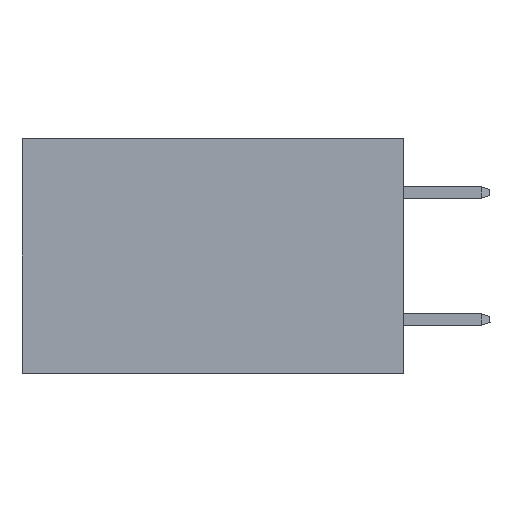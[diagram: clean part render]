
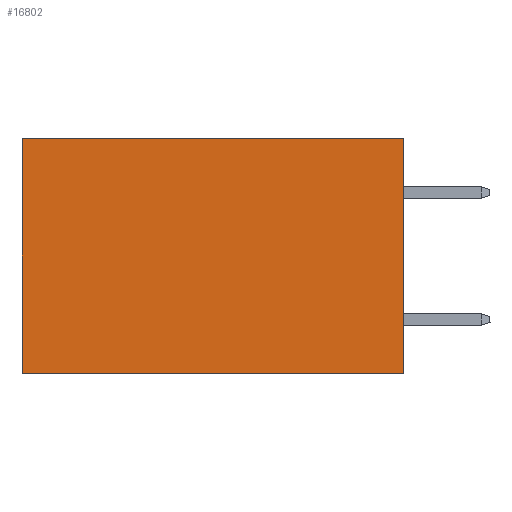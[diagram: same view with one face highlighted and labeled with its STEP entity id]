
A CAD part, left-side view. The second image highlights one B-rep face of the part: STEP entity #16802.
In plain terms, the highlighted planar face has unit normal (-1, 0, 0).
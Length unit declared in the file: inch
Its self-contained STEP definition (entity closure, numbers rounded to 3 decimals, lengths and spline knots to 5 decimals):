
#21 = VECTOR ( 'NONE', #15168, 39.37008 ) ;
#228 = EDGE_CURVE ( 'NONE', #13715, #8388, #10651, .T. ) ;
#1022 = CARTESIAN_POINT ( 'NONE',  ( 0.2875, 0., 0. ) ) ;
#2741 = EDGE_CURVE ( 'NONE', #18579, #13715, #11889, .T. ) ;
#2915 = AXIS2_PLACEMENT_3D ( 'NONE', #3194, #5733, #23075 ) ;
#3194 = CARTESIAN_POINT ( 'NONE',  ( 0.2875, 0., 0. ) ) ;
#3253 = ORIENTED_EDGE ( 'NONE', *, *, #4046, .F. ) ;
#3338 = FACE_OUTER_BOUND ( 'NONE', #24918, .T. ) ;
#4046 = EDGE_CURVE ( 'NONE', #18579, #14857, #15443, .T. ) ;
#5733 = DIRECTION ( 'NONE',  ( 1., 0., 0. ) ) ;
#6467 = DIRECTION ( 'NONE',  ( 0., 0., -1. ) ) ;
#7095 = VECTOR ( 'NONE', #24897, 39.37008 ) ;
#7417 = LINE ( 'NONE', #24339, #7095 ) ;
#8388 = VERTEX_POINT ( 'NONE', #27807 ) ;
#8551 = ORIENTED_EDGE ( 'NONE', *, *, #2741, .T. ) ;
#10651 = LINE ( 'NONE', #15074, #17989 ) ;
#11889 = LINE ( 'NONE', #14150, #18251 ) ;
#13335 = CARTESIAN_POINT ( 'NONE',  ( 0.2875, 0.6, 0. ) ) ;
#13715 = VERTEX_POINT ( 'NONE', #13335 ) ;
#14150 = CARTESIAN_POINT ( 'NONE',  ( 0.2875, 0., 0. ) ) ;
#14857 = VERTEX_POINT ( 'NONE', #17355 ) ;
#15074 = CARTESIAN_POINT ( 'NONE',  ( 0.2875, 0.6, 0. ) ) ;
#15168 = DIRECTION ( 'NONE',  ( 0., 0., -1. ) ) ;
#15443 = LINE ( 'NONE', #21882, #21 ) ;
#16802 = ADVANCED_FACE ( 'NONE', ( #3338 ), #18919, .F. ) ;
#17355 = CARTESIAN_POINT ( 'NONE',  ( 0.2875, 0., -0.37 ) ) ;
#17989 = VECTOR ( 'NONE', #6467, 39.37008 ) ;
#18251 = VECTOR ( 'NONE', #22896, 39.37008 ) ;
#18579 = VERTEX_POINT ( 'NONE', #1022 ) ;
#18919 = PLANE ( 'NONE',  #2915 ) ;
#21034 = EDGE_CURVE ( 'NONE', #14857, #8388, #7417, .T. ) ;
#21882 = CARTESIAN_POINT ( 'NONE',  ( 0.2875, 0., 0. ) ) ;
#22896 = DIRECTION ( 'NONE',  ( 0., 1., 0. ) ) ;
#23075 = DIRECTION ( 'NONE',  ( 0., 0., -1. ) ) ;
#24339 = CARTESIAN_POINT ( 'NONE',  ( 0.2875, 0., -0.37 ) ) ;
#24897 = DIRECTION ( 'NONE',  ( 0., 1., 0. ) ) ;
#24918 = EDGE_LOOP ( 'NONE', ( #25024, #25293, #3253, #8551 ) ) ;
#25024 = ORIENTED_EDGE ( 'NONE', *, *, #228, .T. ) ;
#25293 = ORIENTED_EDGE ( 'NONE', *, *, #21034, .F. ) ;
#27807 = CARTESIAN_POINT ( 'NONE',  ( 0.2875, 0.6, -0.37 ) ) ;
